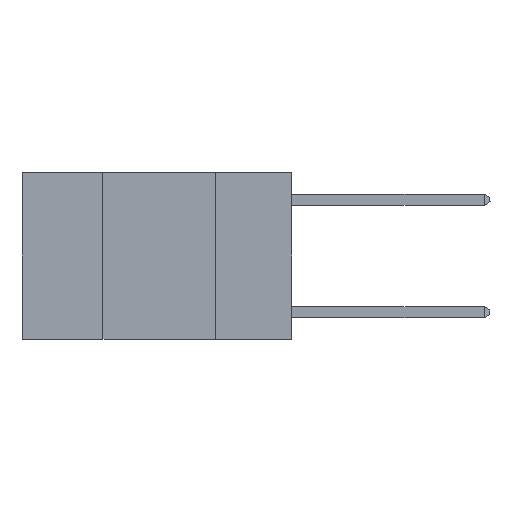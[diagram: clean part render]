
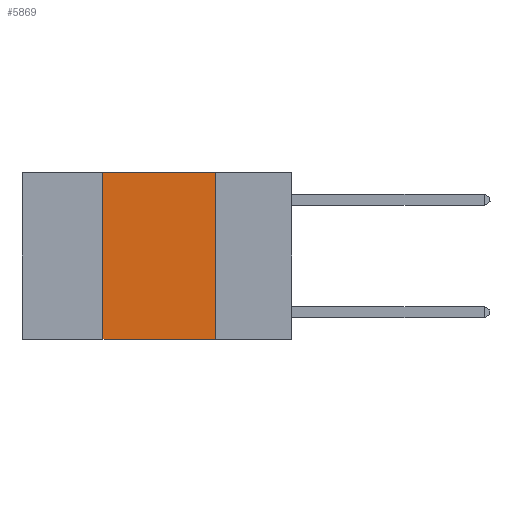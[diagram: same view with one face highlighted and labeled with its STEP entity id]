
A CAD part, left-side view. The second image highlights one B-rep face of the part: STEP entity #5869.
In plain terms, the highlighted planar face has unit normal (-1, 0, 0).
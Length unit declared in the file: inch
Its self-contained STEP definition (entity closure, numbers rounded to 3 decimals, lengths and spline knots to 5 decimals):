
#604 = ORIENTED_EDGE ( 'NONE', *, *, #4073, .F. ) ;
#657 = CARTESIAN_POINT ( 'NONE',  ( 0., 0.42, 0. ) ) ;
#711 = PLANE ( 'NONE',  #5100 ) ;
#852 = LINE ( 'NONE', #7899, #4537 ) ;
#1083 = EDGE_LOOP ( 'NONE', ( #6162, #604, #8196, #6795 ) ) ;
#1247 = VERTEX_POINT ( 'NONE', #8380 ) ;
#1563 = DIRECTION ( 'NONE',  ( 1., 0., 0. ) ) ;
#1961 = VERTEX_POINT ( 'NONE', #4382 ) ;
#2462 = FACE_OUTER_BOUND ( 'NONE', #1083, .T. ) ;
#2508 = CARTESIAN_POINT ( 'NONE',  ( 0., 0.6, -0.37 ) ) ;
#2526 = EDGE_CURVE ( 'NONE', #6125, #1247, #852, .T. ) ;
#2571 = EDGE_CURVE ( 'NONE', #1961, #1247, #9088, .T. ) ;
#2708 = DIRECTION ( 'NONE',  ( 0., 0., 1. ) ) ;
#3542 = EDGE_CURVE ( 'NONE', #1961, #6829, #5159, .T. ) ;
#4073 = EDGE_CURVE ( 'NONE', #6829, #6125, #8265, .T. ) ;
#4382 = CARTESIAN_POINT ( 'NONE',  ( 0., 0.42, -0.37 ) ) ;
#4537 = VECTOR ( 'NONE', #8120, 39.37008 ) ;
#5089 = CARTESIAN_POINT ( 'NONE',  ( 0., 0.6, 0. ) ) ;
#5100 = AXIS2_PLACEMENT_3D ( 'NONE', #5089, #1563, #6455 ) ;
#5159 = LINE ( 'NONE', #7488, #6756 ) ;
#5869 = ADVANCED_FACE ( 'NONE', ( #2462 ), #711, .F. ) ;
#6125 = VERTEX_POINT ( 'NONE', #6569 ) ;
#6162 = ORIENTED_EDGE ( 'NONE', *, *, #2526, .F. ) ;
#6314 = DIRECTION ( 'NONE',  ( 0., -1., 0. ) ) ;
#6455 = DIRECTION ( 'NONE',  ( 0., 0., -1. ) ) ;
#6569 = CARTESIAN_POINT ( 'NONE',  ( 0., 0.17, 0. ) ) ;
#6645 = VECTOR ( 'NONE', #8484, 39.37008 ) ;
#6756 = VECTOR ( 'NONE', #2708, 39.37008 ) ;
#6795 = ORIENTED_EDGE ( 'NONE', *, *, #2571, .T. ) ;
#6829 = VERTEX_POINT ( 'NONE', #657 ) ;
#7319 = VECTOR ( 'NONE', #6314, 39.37008 ) ;
#7488 = CARTESIAN_POINT ( 'NONE',  ( 0., 0.42, 0. ) ) ;
#7839 = CARTESIAN_POINT ( 'NONE',  ( 0., 0.6, 0. ) ) ;
#7899 = CARTESIAN_POINT ( 'NONE',  ( 0., 0.17, 0. ) ) ;
#8120 = DIRECTION ( 'NONE',  ( 0., 0., -1. ) ) ;
#8196 = ORIENTED_EDGE ( 'NONE', *, *, #3542, .F. ) ;
#8265 = LINE ( 'NONE', #7839, #6645 ) ;
#8380 = CARTESIAN_POINT ( 'NONE',  ( 0., 0.17, -0.37 ) ) ;
#8484 = DIRECTION ( 'NONE',  ( 0., -1., 0. ) ) ;
#9088 = LINE ( 'NONE', #2508, #7319 ) ;
